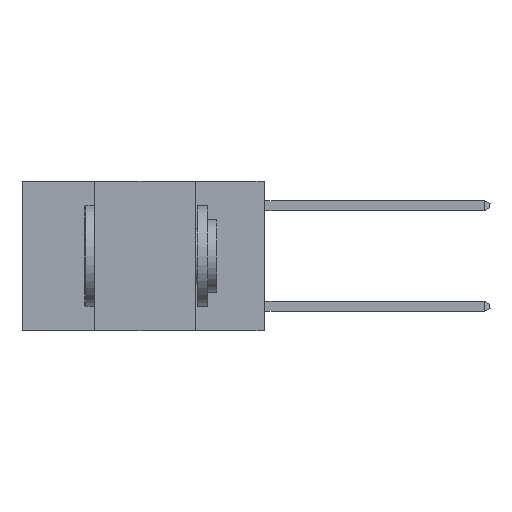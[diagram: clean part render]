
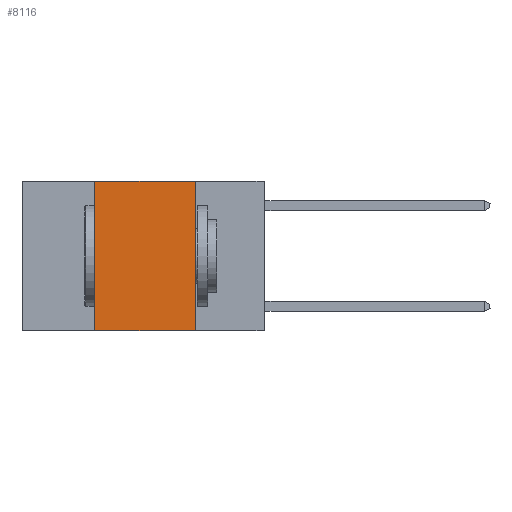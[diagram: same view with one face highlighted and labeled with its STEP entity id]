
A CAD part, left-side view. The second image highlights one B-rep face of the part: STEP entity #8116.
In plain terms, the highlighted planar face has unit normal (-1, 0, 0).
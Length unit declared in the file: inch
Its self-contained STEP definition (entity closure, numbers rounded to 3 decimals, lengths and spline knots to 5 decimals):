
#1159 = AXIS2_PLACEMENT_3D ( 'NONE', #8298, #1852, #7032 ) ;
#1852 = DIRECTION ( 'NONE',  ( 1., 0., 0. ) ) ;
#2772 = VECTOR ( 'NONE', #15541, 39.37008 ) ;
#3364 = EDGE_CURVE ( 'NONE', #7293, #3737, #3528, .T. ) ;
#3528 = LINE ( 'NONE', #4636, #5825 ) ;
#3737 = VERTEX_POINT ( 'NONE', #13425 ) ;
#3845 = EDGE_CURVE ( 'NONE', #11737, #7293, #13832, .T. ) ;
#4122 = LINE ( 'NONE', #10389, #2772 ) ;
#4636 = CARTESIAN_POINT ( 'NONE',  ( 0., 0.17, 0. ) ) ;
#4934 = ORIENTED_EDGE ( 'NONE', *, *, #10366, .F. ) ;
#5362 = ORIENTED_EDGE ( 'NONE', *, *, #3364, .F. ) ;
#5601 = FACE_OUTER_BOUND ( 'NONE', #15169, .T. ) ;
#5817 = CARTESIAN_POINT ( 'NONE',  ( 0., 0.42, -0.37 ) ) ;
#5825 = VECTOR ( 'NONE', #7423, 39.37008 ) ;
#6431 = ORIENTED_EDGE ( 'NONE', *, *, #10047, .T. ) ;
#6754 = ORIENTED_EDGE ( 'NONE', *, *, #3845, .F. ) ;
#7032 = DIRECTION ( 'NONE',  ( 0., 0., -1. ) ) ;
#7293 = VERTEX_POINT ( 'NONE', #8907 ) ;
#7423 = DIRECTION ( 'NONE',  ( 0., 0., -1. ) ) ;
#7987 = VECTOR ( 'NONE', #12163, 39.37008 ) ;
#8116 = ADVANCED_FACE ( 'NONE', ( #5601 ), #16005, .F. ) ;
#8259 = CARTESIAN_POINT ( 'NONE',  ( 0., 0.42, 0. ) ) ;
#8298 = CARTESIAN_POINT ( 'NONE',  ( 0., 0.6, 0. ) ) ;
#8907 = CARTESIAN_POINT ( 'NONE',  ( 0., 0.17, 0. ) ) ;
#9367 = LINE ( 'NONE', #8259, #9768 ) ;
#9768 = VECTOR ( 'NONE', #13439, 39.37008 ) ;
#9871 = CARTESIAN_POINT ( 'NONE',  ( 0., 0.6, 0. ) ) ;
#10047 = EDGE_CURVE ( 'NONE', #14291, #3737, #4122, .T. ) ;
#10366 = EDGE_CURVE ( 'NONE', #14291, #11737, #9367, .T. ) ;
#10389 = CARTESIAN_POINT ( 'NONE',  ( 0., 0.6, -0.37 ) ) ;
#11737 = VERTEX_POINT ( 'NONE', #15411 ) ;
#12163 = DIRECTION ( 'NONE',  ( 0., -1., 0. ) ) ;
#13425 = CARTESIAN_POINT ( 'NONE',  ( 0., 0.17, -0.37 ) ) ;
#13439 = DIRECTION ( 'NONE',  ( 0., 0., 1. ) ) ;
#13832 = LINE ( 'NONE', #9871, #7987 ) ;
#14291 = VERTEX_POINT ( 'NONE', #5817 ) ;
#15169 = EDGE_LOOP ( 'NONE', ( #5362, #6754, #4934, #6431 ) ) ;
#15411 = CARTESIAN_POINT ( 'NONE',  ( 0., 0.42, 0. ) ) ;
#15541 = DIRECTION ( 'NONE',  ( 0., -1., 0. ) ) ;
#16005 = PLANE ( 'NONE',  #1159 ) ;
